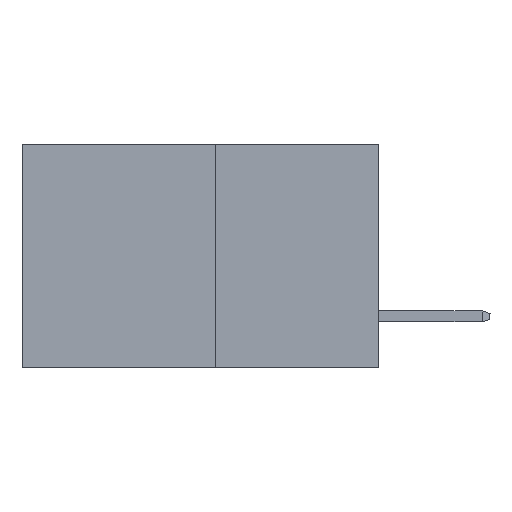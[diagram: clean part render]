
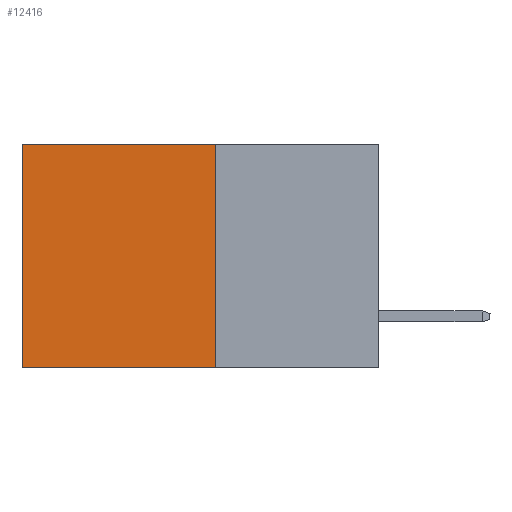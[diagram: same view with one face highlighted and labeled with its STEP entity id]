
A CAD part, left-side view. The second image highlights one B-rep face of the part: STEP entity #12416.
In plain terms, the highlighted planar face has unit normal (-1, 0, 0).
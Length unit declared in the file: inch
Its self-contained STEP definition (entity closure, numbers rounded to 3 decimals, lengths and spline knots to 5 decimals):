
#900 = DIRECTION ( 'NONE',  ( 0., 1., 0. ) ) ;
#1535 = EDGE_CURVE ( 'NONE', #6957, #30612, #5203, .T. ) ;
#2368 = CARTESIAN_POINT ( 'NONE',  ( 0.277, 0.59, 0. ) ) ;
#2423 = FACE_OUTER_BOUND ( 'NONE', #7025, .T. ) ;
#2990 = VECTOR ( 'NONE', #900, 39.37008 ) ;
#4234 = VECTOR ( 'NONE', #23687, 39.37008 ) ;
#5203 = LINE ( 'NONE', #8068, #4234 ) ;
#6429 = CARTESIAN_POINT ( 'NONE',  ( 0.277, 0.59, -0.37 ) ) ;
#6957 = VERTEX_POINT ( 'NONE', #26008 ) ;
#7025 = EDGE_LOOP ( 'NONE', ( #27169, #12603, #12393, #18530 ) ) ;
#7247 = AXIS2_PLACEMENT_3D ( 'NONE', #21055, #13901, #30966 ) ;
#8068 = CARTESIAN_POINT ( 'NONE',  ( 0.277, 0.27, -0.37 ) ) ;
#8876 = EDGE_CURVE ( 'NONE', #27852, #29889, #15292, .T. ) ;
#9525 = CARTESIAN_POINT ( 'NONE',  ( 0.277, 0.27, -0.37 ) ) ;
#9656 = VECTOR ( 'NONE', #11906, 39.37008 ) ;
#11906 = DIRECTION ( 'NONE',  ( 0., 0., -1. ) ) ;
#11920 = DIRECTION ( 'NONE',  ( 0., 1., 0. ) ) ;
#11944 = CARTESIAN_POINT ( 'NONE',  ( 0.277, 0.59, -0.37 ) ) ;
#12393 = ORIENTED_EDGE ( 'NONE', *, *, #1535, .F. ) ;
#12416 = ADVANCED_FACE ( 'NONE', ( #2423 ), #28434, .F. ) ;
#12603 = ORIENTED_EDGE ( 'NONE', *, *, #27213, .F. ) ;
#13901 = DIRECTION ( 'NONE',  ( 1., 0., 0. ) ) ;
#15282 = EDGE_CURVE ( 'NONE', #6957, #27852, #16557, .T. ) ;
#15292 = LINE ( 'NONE', #11944, #9656 ) ;
#16557 = LINE ( 'NONE', #17803, #2990 ) ;
#17803 = CARTESIAN_POINT ( 'NONE',  ( 0.277, 0.27, 0. ) ) ;
#18408 = CARTESIAN_POINT ( 'NONE',  ( 0.277, 0.27, -0.37 ) ) ;
#18530 = ORIENTED_EDGE ( 'NONE', *, *, #15282, .T. ) ;
#21055 = CARTESIAN_POINT ( 'NONE',  ( 0.277, 0.27, -0.37 ) ) ;
#22839 = VECTOR ( 'NONE', #11920, 39.37008 ) ;
#23687 = DIRECTION ( 'NONE',  ( 0., 0., -1. ) ) ;
#26008 = CARTESIAN_POINT ( 'NONE',  ( 0.277, 0.27, 0. ) ) ;
#27169 = ORIENTED_EDGE ( 'NONE', *, *, #8876, .T. ) ;
#27213 = EDGE_CURVE ( 'NONE', #30612, #29889, #29349, .T. ) ;
#27852 = VERTEX_POINT ( 'NONE', #2368 ) ;
#28434 = PLANE ( 'NONE',  #7247 ) ;
#29349 = LINE ( 'NONE', #9525, #22839 ) ;
#29889 = VERTEX_POINT ( 'NONE', #6429 ) ;
#30612 = VERTEX_POINT ( 'NONE', #18408 ) ;
#30966 = DIRECTION ( 'NONE',  ( 0., 0., -1. ) ) ;
